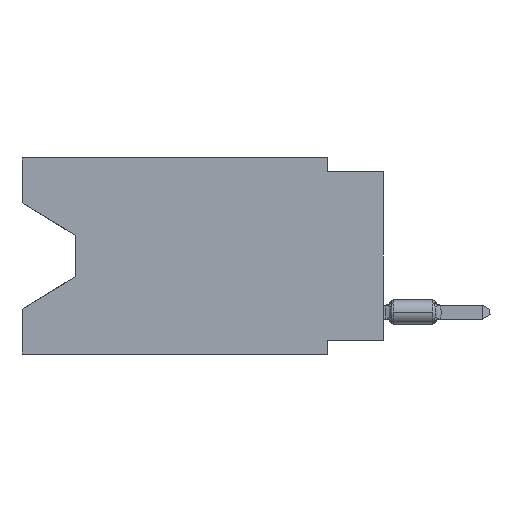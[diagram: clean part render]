
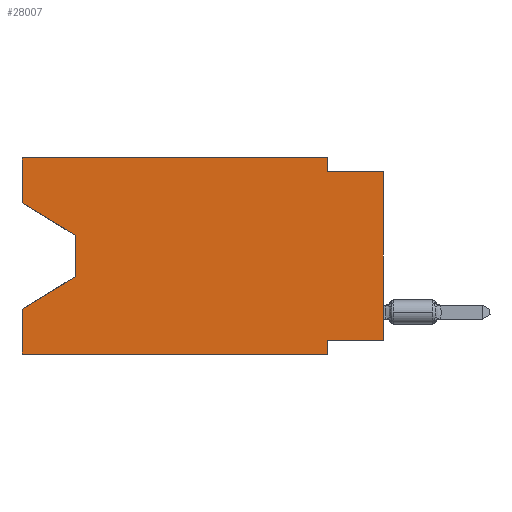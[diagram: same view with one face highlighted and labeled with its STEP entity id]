
A CAD part, left-side view. The second image highlights one B-rep face of the part: STEP entity #28007.
In plain terms, the highlighted planar face has unit normal (-1, 0, 0).
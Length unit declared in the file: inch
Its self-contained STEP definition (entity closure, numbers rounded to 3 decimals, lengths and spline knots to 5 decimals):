
#330 = VECTOR ( 'NONE', #81625, 39.37008 ) ;
#548 = CARTESIAN_POINT ( 'NONE',  ( 0., 0.645, 0. ) ) ;
#1666 = VERTEX_POINT ( 'NONE', #52892 ) ;
#2623 = ORIENTED_EDGE ( 'NONE', *, *, #91902, .F. ) ;
#3087 = VECTOR ( 'NONE', #62376, 39.37008 ) ;
#4518 = VECTOR ( 'NONE', #79775, 39.37008 ) ;
#5179 = DIRECTION ( 'NONE',  ( 0., -0.855, -0.519 ) ) ;
#5422 = CARTESIAN_POINT ( 'NONE',  ( 0., 0.645, -0.35 ) ) ;
#6484 = EDGE_CURVE ( 'NONE', #28582, #47709, #57092, .T. ) ;
#7205 = LINE ( 'NONE', #80807, #73393 ) ;
#8953 = VECTOR ( 'NONE', #73405, 39.37008 ) ;
#12195 = DIRECTION ( 'NONE',  ( 1., 0., 0. ) ) ;
#13144 = CARTESIAN_POINT ( 'NONE',  ( 0., 0.645, 0. ) ) ;
#13585 = VECTOR ( 'NONE', #37510, 39.37008 ) ;
#15907 = CARTESIAN_POINT ( 'NONE',  ( 0., 0.55, -0.212 ) ) ;
#17612 = EDGE_CURVE ( 'NONE', #43043, #1666, #36393, .T. ) ;
#18130 = CARTESIAN_POINT ( 'NONE',  ( 0., 0.55, -0.138 ) ) ;
#18985 = EDGE_CURVE ( 'NONE', #81076, #54247, #7205, .T. ) ;
#19849 = VECTOR ( 'NONE', #44785, 39.37008 ) ;
#20566 = CARTESIAN_POINT ( 'NONE',  ( 0., 0.645, -0.08025 ) ) ;
#21272 = EDGE_CURVE ( 'NONE', #86180, #88398, #73717, .T. ) ;
#22938 = CARTESIAN_POINT ( 'NONE',  ( 0., 0.55, -0.212 ) ) ;
#23173 = EDGE_CURVE ( 'NONE', #47095, #88398, #58118, .T. ) ;
#23522 = ORIENTED_EDGE ( 'NONE', *, *, #23173, .T. ) ;
#24969 = CARTESIAN_POINT ( 'NONE',  ( 0., 0.645, -0.26975 ) ) ;
#26214 = EDGE_CURVE ( 'NONE', #86495, #47709, #30123, .T. ) ;
#27050 = DIRECTION ( 'NONE',  ( 0., -1., 0. ) ) ;
#27486 = CARTESIAN_POINT ( 'NONE',  ( 0., 0.1, -0.025 ) ) ;
#27863 = ORIENTED_EDGE ( 'NONE', *, *, #49317, .T. ) ;
#28007 = ADVANCED_FACE ( 'NONE', ( #48739 ), #78084, .F. ) ;
#28582 = VERTEX_POINT ( 'NONE', #31703 ) ;
#29115 = CARTESIAN_POINT ( 'NONE',  ( 0., 0.1, -0.35 ) ) ;
#29987 = DIRECTION ( 'NONE',  ( 0., -1., 0. ) ) ;
#30123 = LINE ( 'NONE', #22938, #330 ) ;
#31314 = VECTOR ( 'NONE', #63800, 39.37008 ) ;
#31355 = DIRECTION ( 'NONE',  ( 0., -1., 0. ) ) ;
#31703 = CARTESIAN_POINT ( 'NONE',  ( 0., 0.645, -0.35 ) ) ;
#31850 = ORIENTED_EDGE ( 'NONE', *, *, #21272, .F. ) ;
#31884 = CARTESIAN_POINT ( 'NONE',  ( 0., 0.645, 0. ) ) ;
#34710 = VERTEX_POINT ( 'NONE', #80929 ) ;
#34757 = LINE ( 'NONE', #5422, #59517 ) ;
#35708 = VECTOR ( 'NONE', #29987, 39.37008 ) ;
#36320 = ORIENTED_EDGE ( 'NONE', *, *, #18985, .F. ) ;
#36393 = LINE ( 'NONE', #20566, #87812 ) ;
#37510 = DIRECTION ( 'NONE',  ( 0., 0., -1. ) ) ;
#38056 = ORIENTED_EDGE ( 'NONE', *, *, #47555, .F. ) ;
#38644 = LINE ( 'NONE', #31884, #35708 ) ;
#40341 = AXIS2_PLACEMENT_3D ( 'NONE', #13144, #12195, #42472 ) ;
#41187 = CARTESIAN_POINT ( 'NONE',  ( 0., 0.645, -0.08025 ) ) ;
#41657 = LINE ( 'NONE', #70997, #31314 ) ;
#41796 = CARTESIAN_POINT ( 'NONE',  ( 0., 0., 0. ) ) ;
#42472 = DIRECTION ( 'NONE',  ( 0., 0., -1. ) ) ;
#43043 = VERTEX_POINT ( 'NONE', #41187 ) ;
#43774 = CARTESIAN_POINT ( 'NONE',  ( 0., 0.1, 0. ) ) ;
#44785 = DIRECTION ( 'NONE',  ( 0., 0., 1. ) ) ;
#46588 = EDGE_CURVE ( 'NONE', #43043, #34710, #74599, .T. ) ;
#47095 = VERTEX_POINT ( 'NONE', #57848 ) ;
#47555 = EDGE_CURVE ( 'NONE', #50030, #86180, #51954, .T. ) ;
#47709 = VERTEX_POINT ( 'NONE', #24969 ) ;
#48739 = FACE_OUTER_BOUND ( 'NONE', #73868, .T. ) ;
#49317 = EDGE_CURVE ( 'NONE', #1666, #86495, #83563, .T. ) ;
#50030 = VERTEX_POINT ( 'NONE', #79535 ) ;
#51954 = LINE ( 'NONE', #43774, #13585 ) ;
#52892 = CARTESIAN_POINT ( 'NONE',  ( 0., 0.55, -0.138 ) ) ;
#54247 = VERTEX_POINT ( 'NONE', #29115 ) ;
#57092 = LINE ( 'NONE', #71996, #8953 ) ;
#57213 = ORIENTED_EDGE ( 'NONE', *, *, #60913, .T. ) ;
#57848 = CARTESIAN_POINT ( 'NONE',  ( 0., 0., -0.325 ) ) ;
#58118 = LINE ( 'NONE', #41796, #4518 ) ;
#59517 = VECTOR ( 'NONE', #27050, 39.37008 ) ;
#60913 = EDGE_CURVE ( 'NONE', #28582, #54247, #34757, .T. ) ;
#60937 = ORIENTED_EDGE ( 'NONE', *, *, #46588, .F. ) ;
#62376 = DIRECTION ( 'NONE',  ( 0., 0., -1. ) ) ;
#63391 = ORIENTED_EDGE ( 'NONE', *, *, #26214, .T. ) ;
#63800 = DIRECTION ( 'NONE',  ( 0., 1., 0. ) ) ;
#65704 = VECTOR ( 'NONE', #31355, 39.37008 ) ;
#67925 = CARTESIAN_POINT ( 'NONE',  ( 0., 0., -0.025 ) ) ;
#70997 = CARTESIAN_POINT ( 'NONE',  ( 0., 0., -0.325 ) ) ;
#71670 = EDGE_CURVE ( 'NONE', #47095, #81076, #41657, .T. ) ;
#71996 = CARTESIAN_POINT ( 'NONE',  ( 0., 0.645, 0. ) ) ;
#73393 = VECTOR ( 'NONE', #88022, 39.37008 ) ;
#73405 = DIRECTION ( 'NONE',  ( 0., 0., 1. ) ) ;
#73717 = LINE ( 'NONE', #67925, #65704 ) ;
#73868 = EDGE_LOOP ( 'NONE', ( #77485, #27863, #63391, #81598, #57213, #36320, #90738, #23522, #31850, #38056, #2623, #60937 ) ) ;
#74599 = LINE ( 'NONE', #548, #19849 ) ;
#77485 = ORIENTED_EDGE ( 'NONE', *, *, #17612, .T. ) ;
#78084 = PLANE ( 'NONE',  #40341 ) ;
#79535 = CARTESIAN_POINT ( 'NONE',  ( 0., 0.1, 0. ) ) ;
#79775 = DIRECTION ( 'NONE',  ( 0., 0., 1. ) ) ;
#80643 = CARTESIAN_POINT ( 'NONE',  ( 0., 0., -0.025 ) ) ;
#80807 = CARTESIAN_POINT ( 'NONE',  ( 0., 0.1, -0.35 ) ) ;
#80929 = CARTESIAN_POINT ( 'NONE',  ( 0., 0.645, 0. ) ) ;
#81076 = VERTEX_POINT ( 'NONE', #86738 ) ;
#81598 = ORIENTED_EDGE ( 'NONE', *, *, #6484, .F. ) ;
#81625 = DIRECTION ( 'NONE',  ( 0., 0.855, -0.519 ) ) ;
#83563 = LINE ( 'NONE', #18130, #3087 ) ;
#86180 = VERTEX_POINT ( 'NONE', #27486 ) ;
#86495 = VERTEX_POINT ( 'NONE', #15907 ) ;
#86738 = CARTESIAN_POINT ( 'NONE',  ( 0., 0.1, -0.325 ) ) ;
#87812 = VECTOR ( 'NONE', #5179, 39.37008 ) ;
#88022 = DIRECTION ( 'NONE',  ( 0., 0., -1. ) ) ;
#88398 = VERTEX_POINT ( 'NONE', #80643 ) ;
#90738 = ORIENTED_EDGE ( 'NONE', *, *, #71670, .F. ) ;
#91902 = EDGE_CURVE ( 'NONE', #34710, #50030, #38644, .T. ) ;
